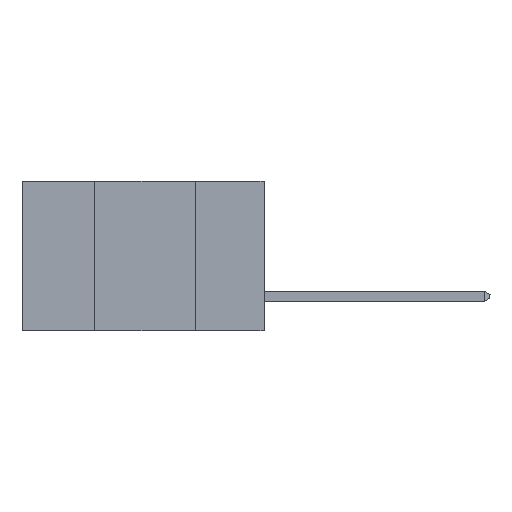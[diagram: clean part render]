
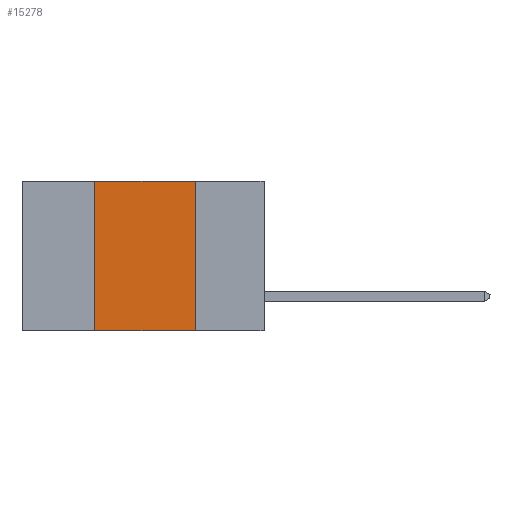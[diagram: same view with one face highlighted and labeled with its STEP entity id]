
A CAD part, left-side view. The second image highlights one B-rep face of the part: STEP entity #15278.
In plain terms, the highlighted planar face has unit normal (-1, 0, 0).
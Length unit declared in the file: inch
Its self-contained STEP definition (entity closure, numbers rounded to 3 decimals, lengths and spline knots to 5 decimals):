
#2523 = EDGE_LOOP ( 'NONE', ( #21839, #7899, #16067, #6735 ) ) ;
#2808 = EDGE_CURVE ( 'NONE', #15011, #24555, #8132, .T. ) ;
#3576 = AXIS2_PLACEMENT_3D ( 'NONE', #19314, #15161, #13524 ) ;
#5864 = VECTOR ( 'NONE', #14126, 39.37008 ) ;
#6735 = ORIENTED_EDGE ( 'NONE', *, *, #2808, .T. ) ;
#7647 = DIRECTION ( 'NONE',  ( 0., -1., 0. ) ) ;
#7899 = ORIENTED_EDGE ( 'NONE', *, *, #19409, .F. ) ;
#8132 = LINE ( 'NONE', #13919, #23974 ) ;
#9163 = LINE ( 'NONE', #11535, #19485 ) ;
#10508 = CARTESIAN_POINT ( 'NONE',  ( 0., 0.17, -0.37 ) ) ;
#11535 = CARTESIAN_POINT ( 'NONE',  ( 0., 0.6, 0. ) ) ;
#12173 = EDGE_CURVE ( 'NONE', #17332, #24555, #18039, .T. ) ;
#13524 = DIRECTION ( 'NONE',  ( 0., 0., -1. ) ) ;
#13912 = CARTESIAN_POINT ( 'NONE',  ( 0., 0.42, -0.37 ) ) ;
#13919 = CARTESIAN_POINT ( 'NONE',  ( 0., 0.6, -0.37 ) ) ;
#14126 = DIRECTION ( 'NONE',  ( 0., 0., -1. ) ) ;
#15011 = VERTEX_POINT ( 'NONE', #13912 ) ;
#15161 = DIRECTION ( 'NONE',  ( 1., 0., 0. ) ) ;
#15278 = ADVANCED_FACE ( 'NONE', ( #17051 ), #24720, .F. ) ;
#15556 = DIRECTION ( 'NONE',  ( 0., -1., 0. ) ) ;
#15914 = VECTOR ( 'NONE', #22723, 39.37008 ) ;
#16067 = ORIENTED_EDGE ( 'NONE', *, *, #23186, .F. ) ;
#16958 = LINE ( 'NONE', #19207, #15914 ) ;
#17051 = FACE_OUTER_BOUND ( 'NONE', #2523, .T. ) ;
#17332 = VERTEX_POINT ( 'NONE', #21415 ) ;
#18039 = LINE ( 'NONE', #19685, #5864 ) ;
#18935 = CARTESIAN_POINT ( 'NONE',  ( 0., 0.42, 0. ) ) ;
#19207 = CARTESIAN_POINT ( 'NONE',  ( 0., 0.42, -0.37 ) ) ;
#19314 = CARTESIAN_POINT ( 'NONE',  ( 0., 0.6, 0. ) ) ;
#19409 = EDGE_CURVE ( 'NONE', #24734, #17332, #9163, .T. ) ;
#19485 = VECTOR ( 'NONE', #7647, 39.37008 ) ;
#19685 = CARTESIAN_POINT ( 'NONE',  ( 0., 0.17, -0.37 ) ) ;
#21415 = CARTESIAN_POINT ( 'NONE',  ( 0., 0.17, 0. ) ) ;
#21839 = ORIENTED_EDGE ( 'NONE', *, *, #12173, .F. ) ;
#22723 = DIRECTION ( 'NONE',  ( 0., 0., 1. ) ) ;
#23186 = EDGE_CURVE ( 'NONE', #15011, #24734, #16958, .T. ) ;
#23974 = VECTOR ( 'NONE', #15556, 39.37008 ) ;
#24555 = VERTEX_POINT ( 'NONE', #10508 ) ;
#24720 = PLANE ( 'NONE',  #3576 ) ;
#24734 = VERTEX_POINT ( 'NONE', #18935 ) ;
